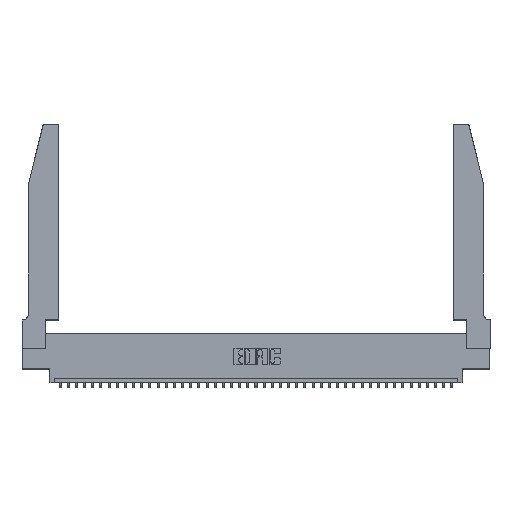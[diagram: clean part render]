
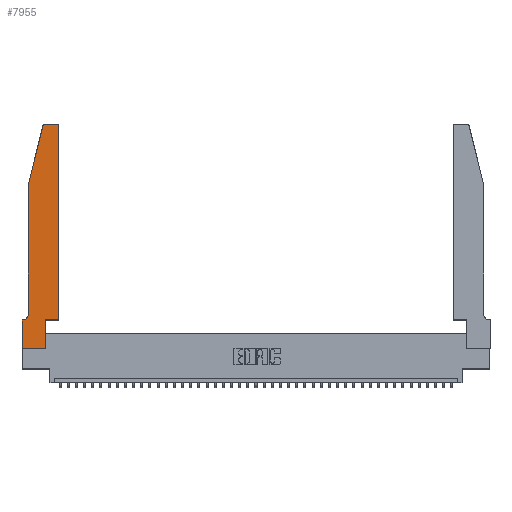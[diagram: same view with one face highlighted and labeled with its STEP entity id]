
A CAD part, top view. The second image highlights one B-rep face of the part: STEP entity #7955.
In plain terms, the highlighted planar face has unit normal (0, 0, 1).
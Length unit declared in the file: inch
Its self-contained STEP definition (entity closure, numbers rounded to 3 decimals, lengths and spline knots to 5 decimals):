
#62 = EDGE_CURVE ( 'NONE', #1098, #9655, #25774, .T. ) ;
#920 = DIRECTION ( 'NONE',  ( 1., 0., 0. ) ) ;
#1098 = VERTEX_POINT ( 'NONE', #25513 ) ;
#2343 = CARTESIAN_POINT ( 'NONE',  ( 0.284, 2.75, 0.37 ) ) ;
#3008 = EDGE_CURVE ( 'NONE', #11248, #27316, #37621, .T. ) ;
#3730 = CARTESIAN_POINT ( 'NONE',  ( 0.0055, 0.35, 0.37 ) ) ;
#4088 = CARTESIAN_POINT ( 'NONE',  ( 0.0755, 2., 0.37 ) ) ;
#4089 = EDGE_CURVE ( 'NONE', #27985, #28013, #17209, .T. ) ;
#5281 = AXIS2_PLACEMENT_3D ( 'NONE', #10413, #32344, #38581 ) ;
#5564 = LINE ( 'NONE', #31608, #36164 ) ;
#5686 = CARTESIAN_POINT ( 'NONE',  ( 0.0755, 2., 0.37 ) ) ;
#6691 = VECTOR ( 'NONE', #9450, 39.37008 ) ;
#6905 = VECTOR ( 'NONE', #13826, 39.37008 ) ;
#7558 = DIRECTION ( 'NONE',  ( 0., -1., 0. ) ) ;
#7955 = ADVANCED_FACE ( 'NONE', ( #11433 ), #39922, .T. ) ;
#8261 = CARTESIAN_POINT ( 'NONE',  ( 0., 0.35, 0.37 ) ) ;
#8493 = AXIS2_PLACEMENT_3D ( 'NONE', #26664, #38953, #26807 ) ;
#8977 = AXIS2_PLACEMENT_3D ( 'NONE', #8261, #33928, #24269 ) ;
#9450 = DIRECTION ( 'NONE',  ( 0., 1., 0. ) ) ;
#9539 = EDGE_CURVE ( 'NONE', #13961, #11248, #32005, .T. ) ;
#9655 = VERTEX_POINT ( 'NONE', #2343 ) ;
#10413 = CARTESIAN_POINT ( 'NONE',  ( 0.284, 2.72, 0.37 ) ) ;
#10477 = EDGE_CURVE ( 'NONE', #37575, #19886, #19567, .T. ) ;
#10488 = ORIENTED_EDGE ( 'NONE', *, *, #21708, .T. ) ;
#10730 = EDGE_CURVE ( 'NONE', #26224, #33736, #40442, .T. ) ;
#10985 = CARTESIAN_POINT ( 'NONE',  ( 0.4505, 0.35, 0.37 ) ) ;
#11248 = VERTEX_POINT ( 'NONE', #26715 ) ;
#11433 = FACE_OUTER_BOUND ( 'NONE', #13058, .T. ) ;
#11884 = ORIENTED_EDGE ( 'NONE', *, *, #9539, .T. ) ;
#12324 = VECTOR ( 'NONE', #33504, 39.37008 ) ;
#12545 = ORIENTED_EDGE ( 'NONE', *, *, #26245, .T. ) ;
#13058 = EDGE_LOOP ( 'NONE', ( #21564, #36569, #38754, #28903, #24678, #25489, #11884, #28717, #10488, #20699, #36943, #12545 ) ) ;
#13418 = VECTOR ( 'NONE', #30586, 39.37008 ) ;
#13799 = CARTESIAN_POINT ( 'NONE',  ( 0.4505, 0.35, 0.37 ) ) ;
#13826 = DIRECTION ( 'NONE',  ( 1., 0., 0. ) ) ;
#13961 = VERTEX_POINT ( 'NONE', #37127 ) ;
#15653 = DIRECTION ( 'NONE',  ( -1., 0., 0. ) ) ;
#16452 = AXIS2_PLACEMENT_3D ( 'NONE', #26330, #32674, #920 ) ;
#17209 = LINE ( 'NONE', #10985, #31556 ) ;
#19567 = CIRCLE ( 'NONE', #8493, 0.07 ) ;
#19886 = VERTEX_POINT ( 'NONE', #3730 ) ;
#20699 = ORIENTED_EDGE ( 'NONE', *, *, #4089, .T. ) ;
#21295 = CIRCLE ( 'NONE', #16452, 0.03 ) ;
#21564 = ORIENTED_EDGE ( 'NONE', *, *, #62, .T. ) ;
#21708 = EDGE_CURVE ( 'NONE', #27316, #27985, #22492, .T. ) ;
#21981 = CARTESIAN_POINT ( 'NONE',  ( 0.2865, 0.35, 0.37 ) ) ;
#22492 = LINE ( 'NONE', #21981, #6691 ) ;
#22593 = VERTEX_POINT ( 'NONE', #30957 ) ;
#24269 = DIRECTION ( 'NONE',  ( 1., 0., 0. ) ) ;
#24320 = EDGE_CURVE ( 'NONE', #19886, #13961, #5564, .T. ) ;
#24678 = ORIENTED_EDGE ( 'NONE', *, *, #10477, .T. ) ;
#25489 = ORIENTED_EDGE ( 'NONE', *, *, #24320, .T. ) ;
#25513 = CARTESIAN_POINT ( 'NONE',  ( 0.4205, 2.75, 0.37 ) ) ;
#25774 = LINE ( 'NONE', #34677, #29740 ) ;
#26224 = VERTEX_POINT ( 'NONE', #36139 ) ;
#26245 = EDGE_CURVE ( 'NONE', #22593, #1098, #21295, .T. ) ;
#26330 = CARTESIAN_POINT ( 'NONE',  ( 0.4205, 2.72, 0.37 ) ) ;
#26664 = CARTESIAN_POINT ( 'NONE',  ( 0.0055, 0.42, 0.37 ) ) ;
#26715 = CARTESIAN_POINT ( 'NONE',  ( 0., 0., 0.37 ) ) ;
#26807 = DIRECTION ( 'NONE',  ( -1., 0., 0. ) ) ;
#27316 = VERTEX_POINT ( 'NONE', #32188 ) ;
#27985 = VERTEX_POINT ( 'NONE', #29675 ) ;
#28013 = VERTEX_POINT ( 'NONE', #13799 ) ;
#28717 = ORIENTED_EDGE ( 'NONE', *, *, #3008, .T. ) ;
#28903 = ORIENTED_EDGE ( 'NONE', *, *, #37651, .T. ) ;
#29675 = CARTESIAN_POINT ( 'NONE',  ( 0.2865, 0.35, 0.37 ) ) ;
#29740 = VECTOR ( 'NONE', #15653, 39.37008 ) ;
#29765 = CIRCLE ( 'NONE', #5281, 0.03 ) ;
#30305 = CARTESIAN_POINT ( 'NONE',  ( 0.4505, 0.35, 0.37 ) ) ;
#30586 = DIRECTION ( 'NONE',  ( 0., 1., 0. ) ) ;
#30957 = CARTESIAN_POINT ( 'NONE',  ( 0.4505, 2.72, 0.37 ) ) ;
#31556 = VECTOR ( 'NONE', #32958, 39.37008 ) ;
#31608 = CARTESIAN_POINT ( 'NONE',  ( 0.0755, 0.35, 0.37 ) ) ;
#31928 = VECTOR ( 'NONE', #40910, 39.37008 ) ;
#32005 = LINE ( 'NONE', #32927, #12324 ) ;
#32050 = EDGE_CURVE ( 'NONE', #28013, #22593, #39661, .T. ) ;
#32188 = CARTESIAN_POINT ( 'NONE',  ( 0.2865, 0., 0.37 ) ) ;
#32344 = DIRECTION ( 'NONE',  ( 0., 0., 1. ) ) ;
#32674 = DIRECTION ( 'NONE',  ( 0., 0., 1. ) ) ;
#32927 = CARTESIAN_POINT ( 'NONE',  ( 0., 0., 0.37 ) ) ;
#32958 = DIRECTION ( 'NONE',  ( 1., 0., 0. ) ) ;
#33504 = DIRECTION ( 'NONE',  ( 0., -1., 0. ) ) ;
#33736 = VERTEX_POINT ( 'NONE', #40042 ) ;
#33928 = DIRECTION ( 'NONE',  ( 0., 0., 1. ) ) ;
#34677 = CARTESIAN_POINT ( 'NONE',  ( 0.2605, 2.75, 0.37 ) ) ;
#35757 = LINE ( 'NONE', #4088, #40767 ) ;
#36139 = CARTESIAN_POINT ( 'NONE',  ( 0.25487, 2.72718, 0.37 ) ) ;
#36164 = VECTOR ( 'NONE', #37592, 39.37008 ) ;
#36569 = ORIENTED_EDGE ( 'NONE', *, *, #40204, .T. ) ;
#36943 = ORIENTED_EDGE ( 'NONE', *, *, #32050, .T. ) ;
#37127 = CARTESIAN_POINT ( 'NONE',  ( 0., 0.35, 0.37 ) ) ;
#37575 = VERTEX_POINT ( 'NONE', #38921 ) ;
#37592 = DIRECTION ( 'NONE',  ( -1., 0., 0. ) ) ;
#37621 = LINE ( 'NONE', #38958, #6905 ) ;
#37651 = EDGE_CURVE ( 'NONE', #33736, #37575, #35757, .T. ) ;
#38581 = DIRECTION ( 'NONE',  ( 1., 0., 0. ) ) ;
#38754 = ORIENTED_EDGE ( 'NONE', *, *, #10730, .T. ) ;
#38921 = CARTESIAN_POINT ( 'NONE',  ( 0.0755, 0.42, 0.37 ) ) ;
#38953 = DIRECTION ( 'NONE',  ( 0., 0., -1. ) ) ;
#38958 = CARTESIAN_POINT ( 'NONE',  ( 0., 0., 0.37 ) ) ;
#39661 = LINE ( 'NONE', #30305, #13418 ) ;
#39922 = PLANE ( 'NONE',  #8977 ) ;
#40042 = CARTESIAN_POINT ( 'NONE',  ( 0.0755, 2., 0.37 ) ) ;
#40204 = EDGE_CURVE ( 'NONE', #9655, #26224, #29765, .T. ) ;
#40442 = LINE ( 'NONE', #5686, #31928 ) ;
#40767 = VECTOR ( 'NONE', #7558, 39.37008 ) ;
#40910 = DIRECTION ( 'NONE',  ( -0.239, -0.971, 0. ) ) ;
